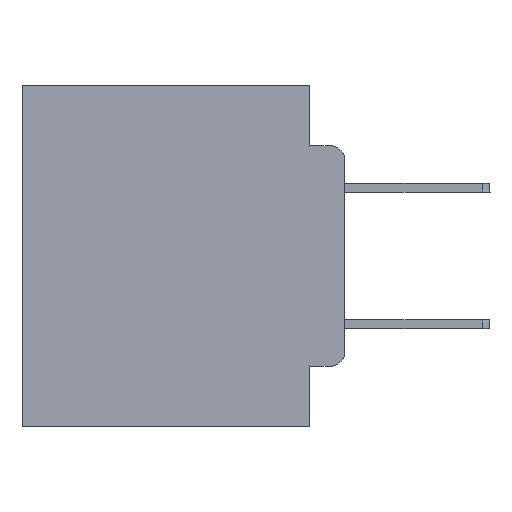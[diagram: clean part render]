
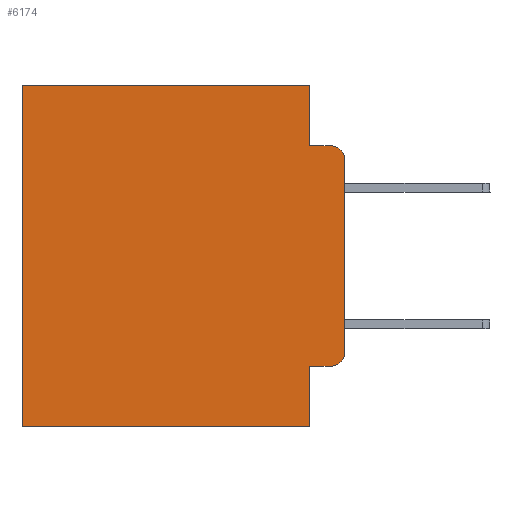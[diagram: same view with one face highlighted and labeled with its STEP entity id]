
A CAD part, left-side view. The second image highlights one B-rep face of the part: STEP entity #6174.
In plain terms, the highlighted planar face has unit normal (-1, 0, 0).
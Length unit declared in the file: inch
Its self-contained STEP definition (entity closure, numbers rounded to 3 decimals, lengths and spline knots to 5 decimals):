
#238 = CARTESIAN_POINT ( 'NONE',  ( 0.298, 0.051, -0.4115 ) ) ;
#1369 = EDGE_CURVE ( 'NONE', #15455, #26682, #9032, .T. ) ;
#1692 = EDGE_CURVE ( 'NONE', #16922, #10366, #23009, .T. ) ;
#1925 = EDGE_LOOP ( 'NONE', ( #26314, #15884, #14950, #11270, #9705, #17296, #16528, #7705, #19326, #18227 ) ) ;
#2031 = VECTOR ( 'NONE', #11102, 39.37008 ) ;
#2190 = CARTESIAN_POINT ( 'NONE',  ( 0.298, 0.051, -0.5 ) ) ;
#2447 = DIRECTION ( 'NONE',  ( 0., 0., -1. ) ) ;
#3527 = VERTEX_POINT ( 'NONE', #19701 ) ;
#6174 = ADVANCED_FACE ( 'NONE', ( #27094 ), #27505, .F. ) ;
#6287 = CIRCLE ( 'NONE', #25929, 0.02 ) ;
#6834 = CARTESIAN_POINT ( 'NONE',  ( 0.298, 0.02, -0.3915 ) ) ;
#7371 = AXIS2_PLACEMENT_3D ( 'NONE', #10129, #16619, #27138 ) ;
#7705 = ORIENTED_EDGE ( 'NONE', *, *, #14913, .F. ) ;
#7808 = CARTESIAN_POINT ( 'NONE',  ( 0.298, 0.02, -0.0885 ) ) ;
#8205 = DIRECTION ( 'NONE',  ( 0., 0., -1. ) ) ;
#8452 = DIRECTION ( 'NONE',  ( 0., 0., -1. ) ) ;
#8991 = DIRECTION ( 'NONE',  ( -1., 0., 0. ) ) ;
#9032 = LINE ( 'NONE', #16821, #14781 ) ;
#9685 = VECTOR ( 'NONE', #23911, 39.37008 ) ;
#9705 = ORIENTED_EDGE ( 'NONE', *, *, #20316, .T. ) ;
#9712 = LINE ( 'NONE', #23173, #24845 ) ;
#10129 = CARTESIAN_POINT ( 'NONE',  ( 0.298, 0., 0. ) ) ;
#10366 = VERTEX_POINT ( 'NONE', #17228 ) ;
#10990 = VERTEX_POINT ( 'NONE', #238 ) ;
#11102 = DIRECTION ( 'NONE',  ( 0., -1., 0. ) ) ;
#11197 = CARTESIAN_POINT ( 'NONE',  ( 0.298, 0.051, -0.4115 ) ) ;
#11270 = ORIENTED_EDGE ( 'NONE', *, *, #23163, .F. ) ;
#12646 = EDGE_CURVE ( 'NONE', #23055, #26299, #22620, .T. ) ;
#13044 = EDGE_CURVE ( 'NONE', #16922, #26682, #23940, .T. ) ;
#13736 = CARTESIAN_POINT ( 'NONE',  ( 0.298, 0.051, -0.0885 ) ) ;
#14699 = VERTEX_POINT ( 'NONE', #15737 ) ;
#14781 = VECTOR ( 'NONE', #18717, 39.37008 ) ;
#14888 = CARTESIAN_POINT ( 'NONE',  ( 0.298, 0., -0.1085 ) ) ;
#14901 = AXIS2_PLACEMENT_3D ( 'NONE', #18844, #25403, #8205 ) ;
#14912 = VECTOR ( 'NONE', #20724, 39.37008 ) ;
#14913 = EDGE_CURVE ( 'NONE', #10990, #20674, #9712, .T. ) ;
#14950 = ORIENTED_EDGE ( 'NONE', *, *, #1369, .F. ) ;
#15080 = VECTOR ( 'NONE', #8452, 39.37008 ) ;
#15289 = EDGE_CURVE ( 'NONE', #20674, #26299, #24144, .T. ) ;
#15455 = VERTEX_POINT ( 'NONE', #13736 ) ;
#15737 = CARTESIAN_POINT ( 'NONE',  ( 0.298, 0.051, 0. ) ) ;
#15884 = ORIENTED_EDGE ( 'NONE', *, *, #13044, .T. ) ;
#15891 = EDGE_CURVE ( 'NONE', #3527, #10366, #6287, .T. ) ;
#15914 = CARTESIAN_POINT ( 'NONE',  ( 0.298, 0., 0. ) ) ;
#16080 = LINE ( 'NONE', #25377, #15080 ) ;
#16375 = CARTESIAN_POINT ( 'NONE',  ( 0.298, 0.473, 0. ) ) ;
#16506 = VECTOR ( 'NONE', #22318, 39.37008 ) ;
#16528 = ORIENTED_EDGE ( 'NONE', *, *, #15289, .F. ) ;
#16619 = DIRECTION ( 'NONE',  ( 1., 0., 0. ) ) ;
#16821 = CARTESIAN_POINT ( 'NONE',  ( 0.298, 0.051, -0.0885 ) ) ;
#16922 = VERTEX_POINT ( 'NONE', #14888 ) ;
#17228 = CARTESIAN_POINT ( 'NONE',  ( 0.298, 0., -0.3915 ) ) ;
#17296 = ORIENTED_EDGE ( 'NONE', *, *, #12646, .T. ) ;
#18227 = ORIENTED_EDGE ( 'NONE', *, *, #15891, .T. ) ;
#18717 = DIRECTION ( 'NONE',  ( 0., -1., 0. ) ) ;
#18844 = CARTESIAN_POINT ( 'NONE',  ( 0.298, 0.02, -0.1085 ) ) ;
#19326 = ORIENTED_EDGE ( 'NONE', *, *, #21490, .T. ) ;
#19701 = CARTESIAN_POINT ( 'NONE',  ( 0.298, 0.02, -0.4115 ) ) ;
#19712 = CARTESIAN_POINT ( 'NONE',  ( 0.298, 0.473, 0. ) ) ;
#19878 = LINE ( 'NONE', #15914, #16506 ) ;
#20316 = EDGE_CURVE ( 'NONE', #14699, #23055, #19878, .T. ) ;
#20674 = VERTEX_POINT ( 'NONE', #2190 ) ;
#20724 = DIRECTION ( 'NONE',  ( 0., 0., -1. ) ) ;
#21490 = EDGE_CURVE ( 'NONE', #10990, #3527, #26262, .T. ) ;
#21781 = DIRECTION ( 'NONE',  ( 0., 0., -1. ) ) ;
#22318 = DIRECTION ( 'NONE',  ( 0., 1., 0. ) ) ;
#22620 = LINE ( 'NONE', #19712, #22992 ) ;
#22992 = VECTOR ( 'NONE', #21781, 39.37008 ) ;
#23009 = LINE ( 'NONE', #26903, #14912 ) ;
#23055 = VERTEX_POINT ( 'NONE', #16375 ) ;
#23163 = EDGE_CURVE ( 'NONE', #14699, #15455, #16080, .T. ) ;
#23173 = CARTESIAN_POINT ( 'NONE',  ( 0.298, 0.051, 0. ) ) ;
#23729 = CARTESIAN_POINT ( 'NONE',  ( 0.298, 0., -0.5 ) ) ;
#23911 = DIRECTION ( 'NONE',  ( 0., 1., 0. ) ) ;
#23940 = CIRCLE ( 'NONE', #14901, 0.02 ) ;
#24144 = LINE ( 'NONE', #23729, #9685 ) ;
#24845 = VECTOR ( 'NONE', #24953, 39.37008 ) ;
#24953 = DIRECTION ( 'NONE',  ( 0., 0., -1. ) ) ;
#25377 = CARTESIAN_POINT ( 'NONE',  ( 0.298, 0.051, 0. ) ) ;
#25403 = DIRECTION ( 'NONE',  ( -1., 0., 0. ) ) ;
#25929 = AXIS2_PLACEMENT_3D ( 'NONE', #6834, #8991, #2447 ) ;
#26124 = CARTESIAN_POINT ( 'NONE',  ( 0.298, 0.473, -0.5 ) ) ;
#26262 = LINE ( 'NONE', #11197, #2031 ) ;
#26299 = VERTEX_POINT ( 'NONE', #26124 ) ;
#26314 = ORIENTED_EDGE ( 'NONE', *, *, #1692, .F. ) ;
#26682 = VERTEX_POINT ( 'NONE', #7808 ) ;
#26903 = CARTESIAN_POINT ( 'NONE',  ( 0.298, 0., 0. ) ) ;
#27094 = FACE_OUTER_BOUND ( 'NONE', #1925, .T. ) ;
#27138 = DIRECTION ( 'NONE',  ( 0., 0., -1. ) ) ;
#27505 = PLANE ( 'NONE',  #7371 ) ;
